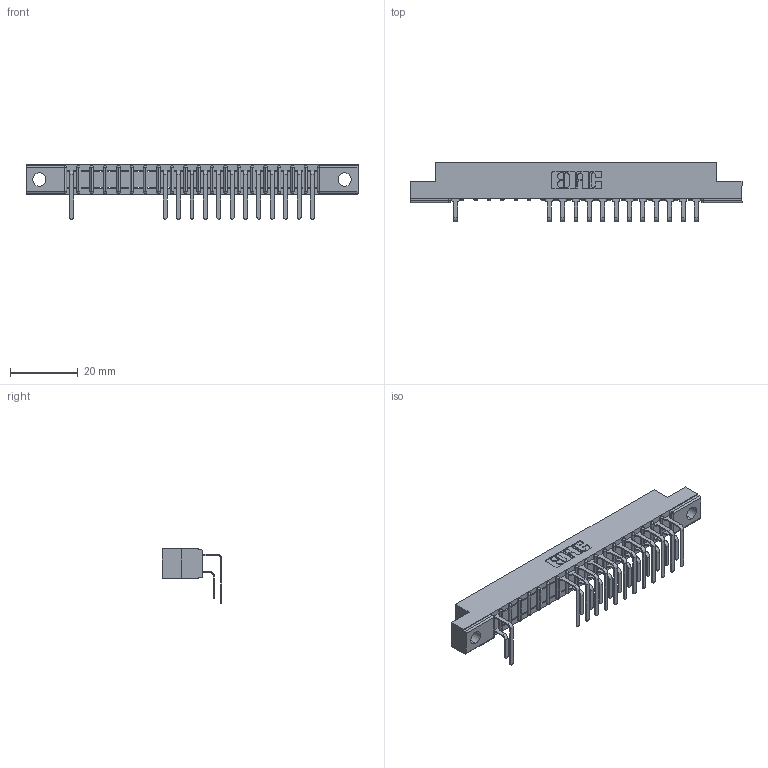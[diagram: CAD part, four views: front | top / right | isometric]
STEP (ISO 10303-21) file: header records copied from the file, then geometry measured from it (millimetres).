
FILE_DESCRIPTION (( 'STEP AP203' ), '1' );
FILE_NAME ('307-038-559-204.STEP', '2018-08-05T12:08:05', ( '' ), ( '' ), 'SwSTEP 2.0', 'SolidWorks 2016', '' );
FILE_SCHEMA (( 'CONFIG_CONTROL_DESIGN' ));
Length unit declared in the file: inch
Products named in the file (4): 307 Part_.156 Dia Mounting Holes; 307-290-001_558 559 - 1 (Single); 307-290-001_559 - 2 (Single); 307-038-559-204
Assembly tree (26 placements, depth 2):
  307-038-559-204
    307 Part_.156 Dia Mounting Holes
    307-290-001_558 559 - 1 (Single)  x12
    307-290-001_559 - 2 (Single)  x13
Bounding box: 98.3 x 17.69 x 16.08 mm (x, y, z)
Volume: 6268.3 mm3; surface area: 10443.2 mm2
Topology: 26 solids, 26 shells, 1532 faces, 4325 edges, 2794 vertices
Faces by surface type: plane 987, cylinder 505, sphere 40
Entity records: 21181 total; most frequent: CARTESIAN_POINT 3534, ORIENTED_EDGE 3510, DIRECTION 3449, EDGE_CURVE 1755, VECTOR 1343, LINE 1343, VERTEX_POINT 1138, AXIS2_PLACEMENT_3D 1053
